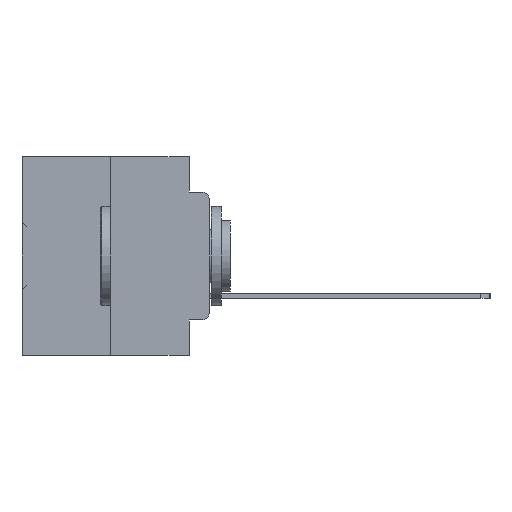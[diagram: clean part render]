
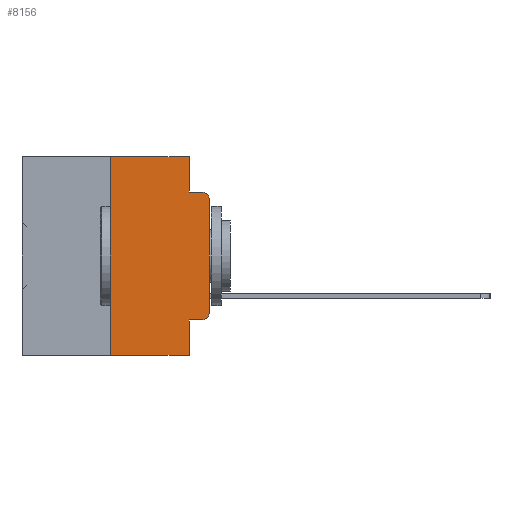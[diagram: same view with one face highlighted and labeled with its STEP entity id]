
A CAD part, left-side view. The second image highlights one B-rep face of the part: STEP entity #8156.
In plain terms, the highlighted planar face has unit normal (-1, 0, 0).
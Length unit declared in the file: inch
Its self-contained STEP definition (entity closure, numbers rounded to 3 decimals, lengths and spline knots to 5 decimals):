
#696 = DIRECTION ( 'NONE',  ( 0., 0., -1. ) ) ;
#1487 = CARTESIAN_POINT ( 'NONE',  ( 0., 0.473, 0. ) ) ;
#2017 = VECTOR ( 'NONE', #18794, 39.37008 ) ;
#2581 = CIRCLE ( 'NONE', #20775, 0.02 ) ;
#2710 = ORIENTED_EDGE ( 'NONE', *, *, #18143, .F. ) ;
#2799 = CARTESIAN_POINT ( 'NONE',  ( 0., 0.051, -0.4115 ) ) ;
#3408 = DIRECTION ( 'NONE',  ( 0., 0., -1. ) ) ;
#3731 = VERTEX_POINT ( 'NONE', #26326 ) ;
#3859 = DIRECTION ( 'NONE',  ( 0., -1., 0. ) ) ;
#4437 = CARTESIAN_POINT ( 'NONE',  ( 0., 0.051, -0.5 ) ) ;
#4567 = EDGE_CURVE ( 'NONE', #13290, #18402, #2581, .T. ) ;
#4979 = ORIENTED_EDGE ( 'NONE', *, *, #24503, .T. ) ;
#6641 = VERTEX_POINT ( 'NONE', #18562 ) ;
#6924 = DIRECTION ( 'NONE',  ( 1., 0., 0. ) ) ;
#8156 = ADVANCED_FACE ( 'NONE', ( #17110 ), #18854, .F. ) ;
#8273 = ORIENTED_EDGE ( 'NONE', *, *, #14588, .F. ) ;
#8543 = EDGE_CURVE ( 'NONE', #6641, #13290, #11967, .T. ) ;
#9408 = VERTEX_POINT ( 'NONE', #22127 ) ;
#9794 = CIRCLE ( 'NONE', #23999, 0.02 ) ;
#10003 = VECTOR ( 'NONE', #24868, 39.37008 ) ;
#10591 = EDGE_CURVE ( 'NONE', #6641, #30413, #28976, .T. ) ;
#11967 = LINE ( 'NONE', #2799, #27732 ) ;
#12008 = VERTEX_POINT ( 'NONE', #33461 ) ;
#13290 = VERTEX_POINT ( 'NONE', #25390 ) ;
#14269 = VECTOR ( 'NONE', #3859, 39.37008 ) ;
#14588 = EDGE_CURVE ( 'NONE', #12008, #18866, #25719, .T. ) ;
#14732 = CARTESIAN_POINT ( 'NONE',  ( 0., 0., -0.3915 ) ) ;
#15265 = EDGE_LOOP ( 'NONE', ( #32477, #4979, #38222, #23635, #2710, #8273, #31991, #25982, #31558, #24586 ) ) ;
#15689 = CARTESIAN_POINT ( 'NONE',  ( 0., 0.25, 0. ) ) ;
#16661 = CARTESIAN_POINT ( 'NONE',  ( 0., 0.02, -0.1085 ) ) ;
#17110 = FACE_OUTER_BOUND ( 'NONE', #15265, .T. ) ;
#18143 = EDGE_CURVE ( 'NONE', #18866, #3731, #26234, .T. ) ;
#18275 = CARTESIAN_POINT ( 'NONE',  ( 0., 0.051, 0. ) ) ;
#18373 = VECTOR ( 'NONE', #25233, 39.37008 ) ;
#18402 = VERTEX_POINT ( 'NONE', #14732 ) ;
#18517 = DIRECTION ( 'NONE',  ( -1., 0., 0. ) ) ;
#18562 = CARTESIAN_POINT ( 'NONE',  ( 0., 0.051, -0.4115 ) ) ;
#18794 = DIRECTION ( 'NONE',  ( 0., 0., 1. ) ) ;
#18854 = PLANE ( 'NONE',  #26330 ) ;
#18866 = VERTEX_POINT ( 'NONE', #34579 ) ;
#19013 = DIRECTION ( 'NONE',  ( 0., -1., 0. ) ) ;
#19532 = LINE ( 'NONE', #33720, #21386 ) ;
#19627 = DIRECTION ( 'NONE',  ( 0., 0., -1. ) ) ;
#20142 = VECTOR ( 'NONE', #27275, 39.37008 ) ;
#20560 = EDGE_CURVE ( 'NONE', #3731, #24613, #22775, .T. ) ;
#20775 = AXIS2_PLACEMENT_3D ( 'NONE', #36131, #18517, #696 ) ;
#21386 = VECTOR ( 'NONE', #19013, 39.37008 ) ;
#22127 = CARTESIAN_POINT ( 'NONE',  ( 0., 0., -0.1085 ) ) ;
#22155 = LINE ( 'NONE', #27544, #14269 ) ;
#22535 = EDGE_CURVE ( 'NONE', #24613, #30960, #22155, .T. ) ;
#22775 = LINE ( 'NONE', #18275, #37464 ) ;
#23597 = DIRECTION ( 'NONE',  ( 0., -1., 0. ) ) ;
#23635 = ORIENTED_EDGE ( 'NONE', *, *, #20560, .F. ) ;
#23999 = AXIS2_PLACEMENT_3D ( 'NONE', #16661, #37237, #19627 ) ;
#24255 = CARTESIAN_POINT ( 'NONE',  ( 0., 0.051, 0. ) ) ;
#24503 = EDGE_CURVE ( 'NONE', #9408, #30960, #9794, .T. ) ;
#24586 = ORIENTED_EDGE ( 'NONE', *, *, #4567, .T. ) ;
#24613 = VERTEX_POINT ( 'NONE', #31919 ) ;
#24785 = CARTESIAN_POINT ( 'NONE',  ( 0., 0.473, 0. ) ) ;
#24868 = DIRECTION ( 'NONE',  ( 0., 0., 1. ) ) ;
#25233 = DIRECTION ( 'NONE',  ( 0., -1., 0. ) ) ;
#25390 = CARTESIAN_POINT ( 'NONE',  ( 0., 0.02, -0.4115 ) ) ;
#25719 = LINE ( 'NONE', #15689, #2017 ) ;
#25982 = ORIENTED_EDGE ( 'NONE', *, *, #10591, .F. ) ;
#26234 = LINE ( 'NONE', #1487, #18373 ) ;
#26326 = CARTESIAN_POINT ( 'NONE',  ( 0., 0.051, 0. ) ) ;
#26330 = AXIS2_PLACEMENT_3D ( 'NONE', #24785, #6924, #27786 ) ;
#27275 = DIRECTION ( 'NONE',  ( 0., 0., -1. ) ) ;
#27544 = CARTESIAN_POINT ( 'NONE',  ( 0., 0.051, -0.0885 ) ) ;
#27732 = VECTOR ( 'NONE', #23597, 39.37008 ) ;
#27786 = DIRECTION ( 'NONE',  ( 0., 0., -1. ) ) ;
#28487 = EDGE_CURVE ( 'NONE', #18402, #9408, #33622, .T. ) ;
#28976 = LINE ( 'NONE', #24255, #20142 ) ;
#30413 = VERTEX_POINT ( 'NONE', #4437 ) ;
#30960 = VERTEX_POINT ( 'NONE', #33589 ) ;
#30998 = EDGE_CURVE ( 'NONE', #12008, #30413, #19532, .T. ) ;
#31558 = ORIENTED_EDGE ( 'NONE', *, *, #8543, .T. ) ;
#31919 = CARTESIAN_POINT ( 'NONE',  ( 0., 0.051, -0.0885 ) ) ;
#31991 = ORIENTED_EDGE ( 'NONE', *, *, #30998, .T. ) ;
#32477 = ORIENTED_EDGE ( 'NONE', *, *, #28487, .T. ) ;
#33461 = CARTESIAN_POINT ( 'NONE',  ( 0., 0.25, -0.5 ) ) ;
#33589 = CARTESIAN_POINT ( 'NONE',  ( 0., 0.02, -0.0885 ) ) ;
#33622 = LINE ( 'NONE', #36554, #10003 ) ;
#33720 = CARTESIAN_POINT ( 'NONE',  ( 0., 0.473, -0.5 ) ) ;
#34579 = CARTESIAN_POINT ( 'NONE',  ( 0., 0.25, 0. ) ) ;
#36131 = CARTESIAN_POINT ( 'NONE',  ( 0., 0.02, -0.3915 ) ) ;
#36554 = CARTESIAN_POINT ( 'NONE',  ( 0., 0., 0. ) ) ;
#37237 = DIRECTION ( 'NONE',  ( -1., 0., 0. ) ) ;
#37464 = VECTOR ( 'NONE', #3408, 39.37008 ) ;
#38222 = ORIENTED_EDGE ( 'NONE', *, *, #22535, .F. ) ;
